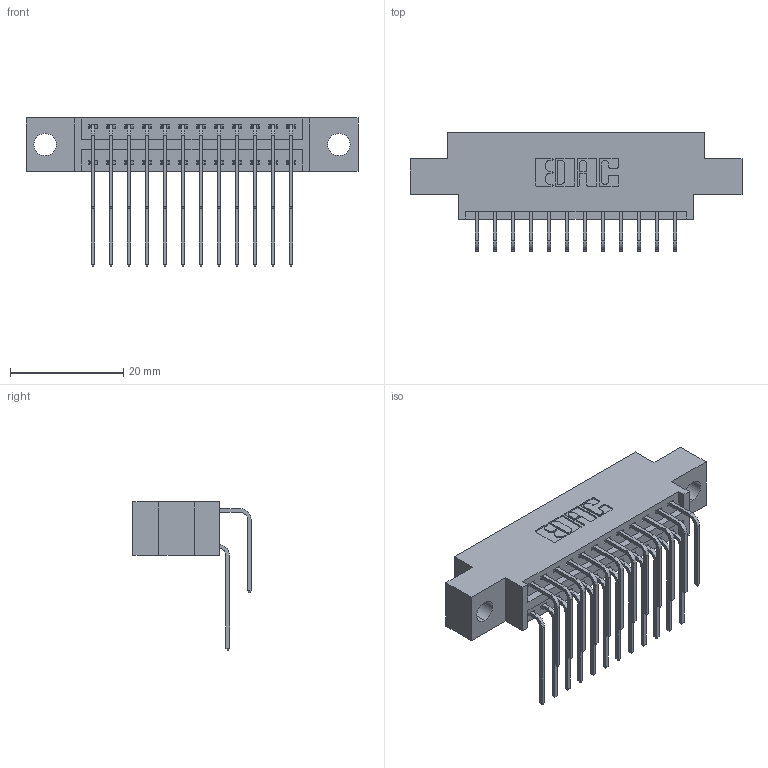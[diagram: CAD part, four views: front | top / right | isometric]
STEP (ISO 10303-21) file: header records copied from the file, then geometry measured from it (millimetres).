
FILE_DESCRIPTION (( 'STEP AP203' ), '1' );
FILE_NAME ('346-024-559-804.STEP', '2022-05-19T00:32:31', ( '' ), ( '' ), 'SwSTEP 2.0', 'SolidWorks 2020', '' );
FILE_SCHEMA (( 'CONFIG_CONTROL_DESIGN' ));
Length unit declared in the file: inch
Products named in the file (4): 346-024-559-804; 346 Part_0.170 Offset - 0.156 Dia-TH; 345-292-001_558 559 Tail - 1; 345-292-001_559 Tail - 2
Assembly tree (25 placements, depth 2):
  346-024-559-804
    346 Part_0.170 Offset - 0.156 Dia-TH
    345-292-001_558 559 Tail - 1  x12
    345-292-001_559 Tail - 2  x12
Bounding box: 58.67 x 20.89 x 26.16 mm (x, y, z)
Volume: 5366.3 mm3; surface area: 7596.6 mm2
Topology: 25 solids, 25 shells, 1436 faces, 4241 edges, 2794 vertices
Faces by surface type: plane 982, cylinder 454
Entity records: 14205 total; most frequent: CARTESIAN_POINT 2441, ORIENTED_EDGE 2322, DIRECTION 2173, EDGE_CURVE 1161, LINE 941, VECTOR 941, VERTEX_POINT 770, AXIS2_PLACEMENT_3D 616
